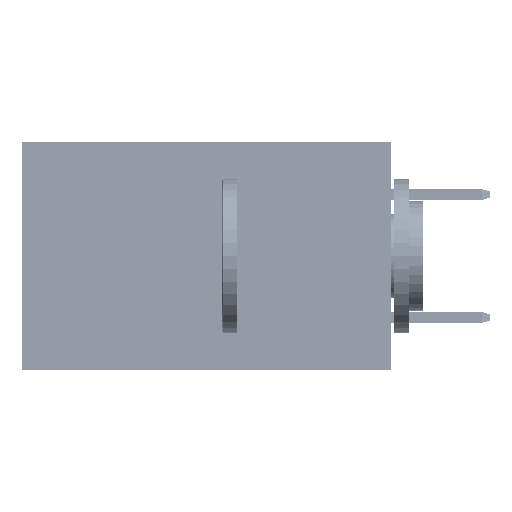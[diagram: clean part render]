
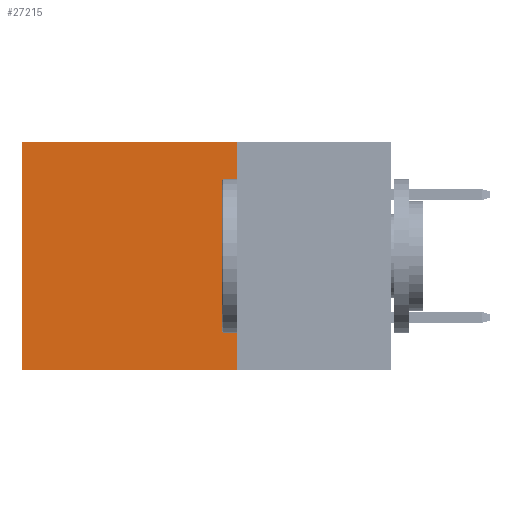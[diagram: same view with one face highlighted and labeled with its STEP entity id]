
A CAD part, left-side view. The second image highlights one B-rep face of the part: STEP entity #27215.
In plain terms, the highlighted planar face has unit normal (-1, 0, 0).
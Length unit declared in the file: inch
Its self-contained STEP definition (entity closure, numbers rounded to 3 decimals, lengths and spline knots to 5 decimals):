
#91 = DIRECTION ( 'NONE',  ( 0., 1., 0. ) ) ;
#196 = VERTEX_POINT ( 'NONE', #20419 ) ;
#873 = CARTESIAN_POINT ( 'NONE',  ( 0.2875, 0.25, 0. ) ) ;
#2141 = DIRECTION ( 'NONE',  ( 0., 0., -1. ) ) ;
#4072 = VECTOR ( 'NONE', #91, 39.37008 ) ;
#7382 = EDGE_CURVE ( 'NONE', #45653, #24360, #23821, .T. ) ;
#8319 = EDGE_LOOP ( 'NONE', ( #15154, #47625, #18505, #24767 ) ) ;
#9744 = CARTESIAN_POINT ( 'NONE',  ( 0.2875, 0.25, 0. ) ) ;
#10215 = CARTESIAN_POINT ( 'NONE',  ( 0.2875, 0.25, 0. ) ) ;
#10751 = LINE ( 'NONE', #12349, #38577 ) ;
#12349 = CARTESIAN_POINT ( 'NONE',  ( 0.2875, 0.6, 0. ) ) ;
#15154 = ORIENTED_EDGE ( 'NONE', *, *, #27570, .T. ) ;
#18505 = ORIENTED_EDGE ( 'NONE', *, *, #20024, .F. ) ;
#19344 = CARTESIAN_POINT ( 'NONE',  ( 0.2875, 0.25, -0.37 ) ) ;
#19364 = CARTESIAN_POINT ( 'NONE',  ( 0.2875, 0.6, -0.37 ) ) ;
#20024 = EDGE_CURVE ( 'NONE', #45653, #196, #31988, .T. ) ;
#20419 = CARTESIAN_POINT ( 'NONE',  ( 0.2875, 0.25, -0.37 ) ) ;
#21958 = VECTOR ( 'NONE', #36873, 39.37008 ) ;
#23821 = LINE ( 'NONE', #873, #32666 ) ;
#24360 = VERTEX_POINT ( 'NONE', #34579 ) ;
#24767 = ORIENTED_EDGE ( 'NONE', *, *, #7382, .T. ) ;
#25133 = DIRECTION ( 'NONE',  ( 1., 0., 0. ) ) ;
#27215 = ADVANCED_FACE ( 'NONE', ( #43951 ), #32576, .F. ) ;
#27448 = EDGE_CURVE ( 'NONE', #196, #35361, #34473, .T. ) ;
#27570 = EDGE_CURVE ( 'NONE', #24360, #35361, #10751, .T. ) ;
#30671 = AXIS2_PLACEMENT_3D ( 'NONE', #40120, #25133, #2141 ) ;
#31988 = LINE ( 'NONE', #10215, #21958 ) ;
#32576 = PLANE ( 'NONE',  #30671 ) ;
#32666 = VECTOR ( 'NONE', #38864, 39.37008 ) ;
#34473 = LINE ( 'NONE', #19344, #4072 ) ;
#34579 = CARTESIAN_POINT ( 'NONE',  ( 0.2875, 0.6, 0. ) ) ;
#35361 = VERTEX_POINT ( 'NONE', #19364 ) ;
#36873 = DIRECTION ( 'NONE',  ( 0., 0., -1. ) ) ;
#38577 = VECTOR ( 'NONE', #42620, 39.37008 ) ;
#38864 = DIRECTION ( 'NONE',  ( 0., 1., 0. ) ) ;
#40120 = CARTESIAN_POINT ( 'NONE',  ( 0.2875, 0.25, 0. ) ) ;
#42620 = DIRECTION ( 'NONE',  ( 0., 0., -1. ) ) ;
#43951 = FACE_OUTER_BOUND ( 'NONE', #8319, .T. ) ;
#45653 = VERTEX_POINT ( 'NONE', #9744 ) ;
#47625 = ORIENTED_EDGE ( 'NONE', *, *, #27448, .F. ) ;
